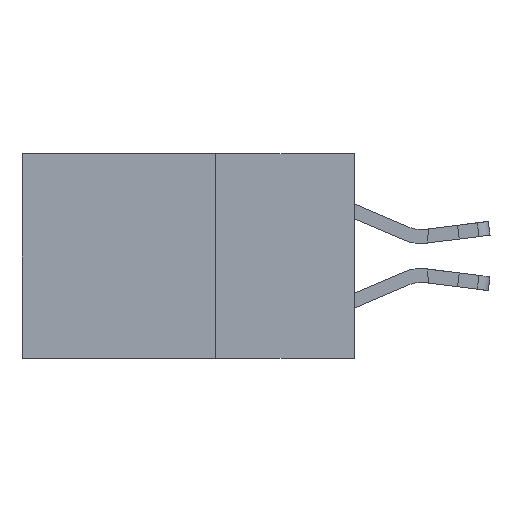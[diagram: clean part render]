
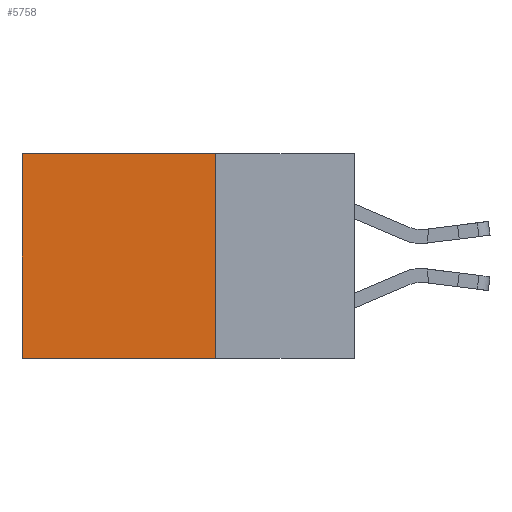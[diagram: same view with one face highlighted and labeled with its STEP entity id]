
A CAD part, left-side view. The second image highlights one B-rep face of the part: STEP entity #5758.
In plain terms, the highlighted planar face has unit normal (-1, 0, 0).
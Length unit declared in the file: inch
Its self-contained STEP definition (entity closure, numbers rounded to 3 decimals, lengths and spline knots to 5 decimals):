
#73 = VERTEX_POINT ( 'NONE', #10324 ) ;
#167 = LINE ( 'NONE', #4701, #2305 ) ;
#204 = EDGE_CURVE ( 'NONE', #2091, #5774, #7757, .T. ) ;
#451 = CARTESIAN_POINT ( 'NONE',  ( 0.2615, 0.6, 0. ) ) ;
#842 = CARTESIAN_POINT ( 'NONE',  ( 0.2615, 0.25, -0.37 ) ) ;
#1032 = DIRECTION ( 'NONE',  ( 0., 1., 0. ) ) ;
#1203 = ORIENTED_EDGE ( 'NONE', *, *, #8453, .F. ) ;
#1607 = EDGE_CURVE ( 'NONE', #6130, #2091, #4202, .T. ) ;
#2020 = EDGE_LOOP ( 'NONE', ( #3275, #6834, #1203, #8779 ) ) ;
#2091 = VERTEX_POINT ( 'NONE', #451 ) ;
#2305 = VECTOR ( 'NONE', #1032, 39.37008 ) ;
#2488 = DIRECTION ( 'NONE',  ( 0., 0., -1. ) ) ;
#2543 = VECTOR ( 'NONE', #9701, 39.37008 ) ;
#3275 = ORIENTED_EDGE ( 'NONE', *, *, #204, .T. ) ;
#4202 = LINE ( 'NONE', #6314, #5288 ) ;
#4511 = CARTESIAN_POINT ( 'NONE',  ( 0.2615, 0.25, -0.37 ) ) ;
#4701 = CARTESIAN_POINT ( 'NONE',  ( 0.2615, 0.25, -0.37 ) ) ;
#5256 = CARTESIAN_POINT ( 'NONE',  ( 0.2615, 0.6, -0.37 ) ) ;
#5288 = VECTOR ( 'NONE', #6248, 39.37008 ) ;
#5758 = ADVANCED_FACE ( 'NONE', ( #7219 ), #8139, .F. ) ;
#5774 = VERTEX_POINT ( 'NONE', #5256 ) ;
#6130 = VERTEX_POINT ( 'NONE', #6849 ) ;
#6248 = DIRECTION ( 'NONE',  ( 0., 1., 0. ) ) ;
#6314 = CARTESIAN_POINT ( 'NONE',  ( 0.2615, 0.25, 0. ) ) ;
#6721 = CARTESIAN_POINT ( 'NONE',  ( 0.2615, 0.6, -0.37 ) ) ;
#6834 = ORIENTED_EDGE ( 'NONE', *, *, #8614, .F. ) ;
#6849 = CARTESIAN_POINT ( 'NONE',  ( 0.2615, 0.25, 0. ) ) ;
#7219 = FACE_OUTER_BOUND ( 'NONE', #2020, .T. ) ;
#7757 = LINE ( 'NONE', #6721, #2543 ) ;
#8139 = PLANE ( 'NONE',  #10092 ) ;
#8453 = EDGE_CURVE ( 'NONE', #6130, #73, #9623, .T. ) ;
#8614 = EDGE_CURVE ( 'NONE', #73, #5774, #167, .T. ) ;
#8779 = ORIENTED_EDGE ( 'NONE', *, *, #1607, .T. ) ;
#9556 = VECTOR ( 'NONE', #2488, 39.37008 ) ;
#9623 = LINE ( 'NONE', #842, #9556 ) ;
#9701 = DIRECTION ( 'NONE',  ( 0., 0., -1. ) ) ;
#10092 = AXIS2_PLACEMENT_3D ( 'NONE', #4511, #10829, #11688 ) ;
#10324 = CARTESIAN_POINT ( 'NONE',  ( 0.2615, 0.25, -0.37 ) ) ;
#10829 = DIRECTION ( 'NONE',  ( 1., 0., 0. ) ) ;
#11688 = DIRECTION ( 'NONE',  ( 0., 0., -1. ) ) ;
